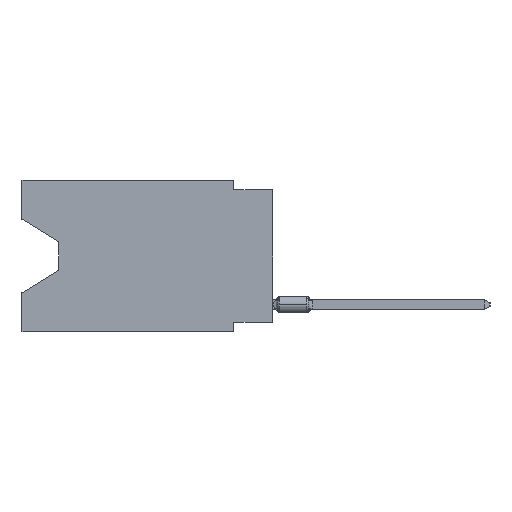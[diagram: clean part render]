
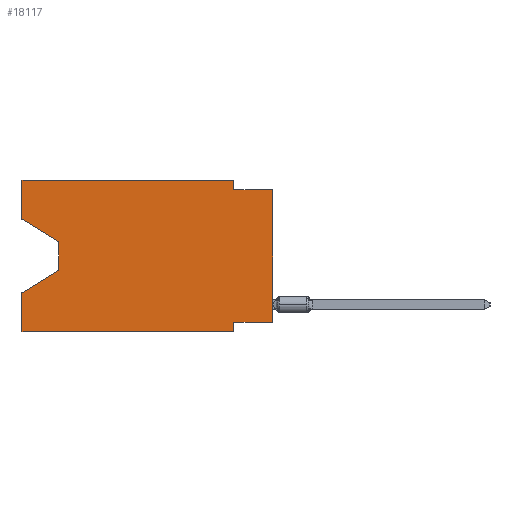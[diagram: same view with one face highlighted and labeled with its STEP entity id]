
A CAD part, left-side view. The second image highlights one B-rep face of the part: STEP entity #18117.
In plain terms, the highlighted planar face has unit normal (-1, 0, 0).
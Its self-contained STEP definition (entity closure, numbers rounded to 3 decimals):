
#371 = VECTOR ( 'NONE', #14272, 1000. ) ;
#644 = EDGE_CURVE ( 'NONE', #26634, #58440, #25595, .T. ) ;
#842 = AXIS2_PLACEMENT_3D ( 'NONE', #12866, #32668, #27325 ) ;
#1471 = CARTESIAN_POINT ( 'NONE',  ( 0., 16.383, -7.36 ) ) ;
#3089 = VECTOR ( 'NONE', #30066, 1000. ) ;
#4349 = LINE ( 'NONE', #53198, #32347 ) ;
#4712 = FACE_OUTER_BOUND ( 'NONE', #42978, .T. ) ;
#4806 = DIRECTION ( 'NONE',  ( 0., 0., -1. ) ) ;
#5426 = CARTESIAN_POINT ( 'NONE',  ( 0., 0., -9.271 ) ) ;
#5575 = CARTESIAN_POINT ( 'NONE',  ( 0., 2.54, 0. ) ) ;
#7225 = VERTEX_POINT ( 'NONE', #35555 ) ;
#7601 = ORIENTED_EDGE ( 'NONE', *, *, #14085, .T. ) ;
#8124 = DIRECTION ( 'NONE',  ( 0., -1., 0. ) ) ;
#8174 = PLANE ( 'NONE',  #842 ) ;
#9538 = ORIENTED_EDGE ( 'NONE', *, *, #37400, .T. ) ;
#10164 = CARTESIAN_POINT ( 'NONE',  ( 0., 16.383, -2.546 ) ) ;
#10740 = DIRECTION ( 'NONE',  ( 0., 1., 0. ) ) ;
#11136 = CARTESIAN_POINT ( 'NONE',  ( 0., 16.383, 0. ) ) ;
#12228 = CARTESIAN_POINT ( 'NONE',  ( 0., 0., -0.635 ) ) ;
#12586 = DIRECTION ( 'NONE',  ( 0., 0., 1. ) ) ;
#12726 = EDGE_CURVE ( 'NONE', #24708, #59375, #4349, .T. ) ;
#12866 = CARTESIAN_POINT ( 'NONE',  ( 0., 16.383, 0. ) ) ;
#13917 = EDGE_CURVE ( 'NONE', #58440, #14348, #37642, .T. ) ;
#14085 = EDGE_CURVE ( 'NONE', #29590, #41912, #17613, .T. ) ;
#14195 = ORIENTED_EDGE ( 'NONE', *, *, #21123, .F. ) ;
#14272 = DIRECTION ( 'NONE',  ( 0., 0., 1. ) ) ;
#14348 = VERTEX_POINT ( 'NONE', #1471 ) ;
#14440 = DIRECTION ( 'NONE',  ( 0., -1., 0. ) ) ;
#14739 = CARTESIAN_POINT ( 'NONE',  ( 0., 16.383, -9.906 ) ) ;
#16146 = VERTEX_POINT ( 'NONE', #43399 ) ;
#17130 = CARTESIAN_POINT ( 'NONE',  ( 0., 16.383, 0. ) ) ;
#17613 = LINE ( 'NONE', #21090, #21535 ) ;
#18117 = ADVANCED_FACE ( 'NONE', ( #4712 ), #8174, .F. ) ;
#20408 = DIRECTION ( 'NONE',  ( 0., -1., 0. ) ) ;
#20557 = LINE ( 'NONE', #11136, #42137 ) ;
#21090 = CARTESIAN_POINT ( 'NONE',  ( 0., 0., 0. ) ) ;
#21123 = EDGE_CURVE ( 'NONE', #36607, #16146, #52195, .T. ) ;
#21336 = CARTESIAN_POINT ( 'NONE',  ( 0., 0., -0.635 ) ) ;
#21535 = VECTOR ( 'NONE', #12586, 1000. ) ;
#21788 = EDGE_CURVE ( 'NONE', #53123, #16146, #57440, .T. ) ;
#23298 = EDGE_CURVE ( 'NONE', #29590, #36607, #24888, .T. ) ;
#23351 = VECTOR ( 'NONE', #10740, 1000. ) ;
#23691 = LINE ( 'NONE', #10164, #24199 ) ;
#24199 = VECTOR ( 'NONE', #42536, 1000. ) ;
#24708 = VERTEX_POINT ( 'NONE', #17130 ) ;
#24866 = ORIENTED_EDGE ( 'NONE', *, *, #644, .T. ) ;
#24888 = LINE ( 'NONE', #5426, #23351 ) ;
#25595 = LINE ( 'NONE', #59791, #47453 ) ;
#26134 = VECTOR ( 'NONE', #4806, 1000. ) ;
#26634 = VERTEX_POINT ( 'NONE', #56807 ) ;
#26895 = EDGE_CURVE ( 'NONE', #53123, #14348, #32199, .T. ) ;
#27176 = VERTEX_POINT ( 'NONE', #51252 ) ;
#27247 = CARTESIAN_POINT ( 'NONE',  ( 0., 2.54, -9.271 ) ) ;
#27325 = DIRECTION ( 'NONE',  ( 0., 0., -1. ) ) ;
#27735 = CARTESIAN_POINT ( 'NONE',  ( 0., 2.54, -9.906 ) ) ;
#29223 = VECTOR ( 'NONE', #14440, 1000. ) ;
#29590 = VERTEX_POINT ( 'NONE', #44000 ) ;
#30066 = DIRECTION ( 'NONE',  ( 0., 0., -1. ) ) ;
#32199 = LINE ( 'NONE', #56661, #371 ) ;
#32347 = VECTOR ( 'NONE', #8124, 1000. ) ;
#32626 = CARTESIAN_POINT ( 'NONE',  ( 0., 13.97, -5.893 ) ) ;
#32668 = DIRECTION ( 'NONE',  ( 1., 0., 0. ) ) ;
#34395 = DIRECTION ( 'NONE',  ( 0., 0., 1. ) ) ;
#34423 = CARTESIAN_POINT ( 'NONE',  ( 0., 2.54, 0. ) ) ;
#35555 = CARTESIAN_POINT ( 'NONE',  ( 0., 2.54, -0.635 ) ) ;
#36162 = ORIENTED_EDGE ( 'NONE', *, *, #46485, .F. ) ;
#36215 = ORIENTED_EDGE ( 'NONE', *, *, #46785, .F. ) ;
#36607 = VERTEX_POINT ( 'NONE', #27247 ) ;
#37400 = EDGE_CURVE ( 'NONE', #27176, #26634, #23691, .T. ) ;
#37642 = LINE ( 'NONE', #32626, #52626 ) ;
#40347 = ORIENTED_EDGE ( 'NONE', *, *, #43925, .F. ) ;
#41092 = ORIENTED_EDGE ( 'NONE', *, *, #26895, .F. ) ;
#41912 = VERTEX_POINT ( 'NONE', #12228 ) ;
#42137 = VECTOR ( 'NONE', #34395, 1000. ) ;
#42536 = DIRECTION ( 'NONE',  ( 0., -0.855, -0.519 ) ) ;
#42978 = EDGE_LOOP ( 'NONE', ( #9538, #24866, #56056, #41092, #44608, #14195, #55762, #7601, #40347, #36215, #54437, #36162 ) ) ;
#43367 = CARTESIAN_POINT ( 'NONE',  ( 0., 13.97, -5.893 ) ) ;
#43399 = CARTESIAN_POINT ( 'NONE',  ( 0., 2.54, -9.906 ) ) ;
#43925 = EDGE_CURVE ( 'NONE', #7225, #41912, #49900, .T. ) ;
#44000 = CARTESIAN_POINT ( 'NONE',  ( 0., 0., -9.271 ) ) ;
#44608 = ORIENTED_EDGE ( 'NONE', *, *, #21788, .T. ) ;
#44959 = VECTOR ( 'NONE', #20408, 1000. ) ;
#45609 = CARTESIAN_POINT ( 'NONE',  ( 0., 16.383, -9.906 ) ) ;
#46485 = EDGE_CURVE ( 'NONE', #27176, #24708, #20557, .T. ) ;
#46785 = EDGE_CURVE ( 'NONE', #59375, #7225, #53269, .T. ) ;
#47061 = DIRECTION ( 'NONE',  ( 0., 0.855, -0.519 ) ) ;
#47453 = VECTOR ( 'NONE', #54757, 1000. ) ;
#49900 = LINE ( 'NONE', #21336, #44959 ) ;
#51252 = CARTESIAN_POINT ( 'NONE',  ( 0., 16.383, -2.546 ) ) ;
#52195 = LINE ( 'NONE', #27735, #26134 ) ;
#52626 = VECTOR ( 'NONE', #47061, 1000. ) ;
#53123 = VERTEX_POINT ( 'NONE', #45609 ) ;
#53198 = CARTESIAN_POINT ( 'NONE',  ( 0., 16.383, 0. ) ) ;
#53269 = LINE ( 'NONE', #5575, #3089 ) ;
#54437 = ORIENTED_EDGE ( 'NONE', *, *, #12726, .F. ) ;
#54757 = DIRECTION ( 'NONE',  ( 0., 0., -1. ) ) ;
#55762 = ORIENTED_EDGE ( 'NONE', *, *, #23298, .F. ) ;
#56056 = ORIENTED_EDGE ( 'NONE', *, *, #13917, .T. ) ;
#56661 = CARTESIAN_POINT ( 'NONE',  ( 0., 16.383, 0. ) ) ;
#56807 = CARTESIAN_POINT ( 'NONE',  ( 0., 13.97, -4.013 ) ) ;
#57440 = LINE ( 'NONE', #14739, #29223 ) ;
#58440 = VERTEX_POINT ( 'NONE', #43367 ) ;
#59375 = VERTEX_POINT ( 'NONE', #34423 ) ;
#59791 = CARTESIAN_POINT ( 'NONE',  ( 0., 13.97, -4.013 ) ) ;
